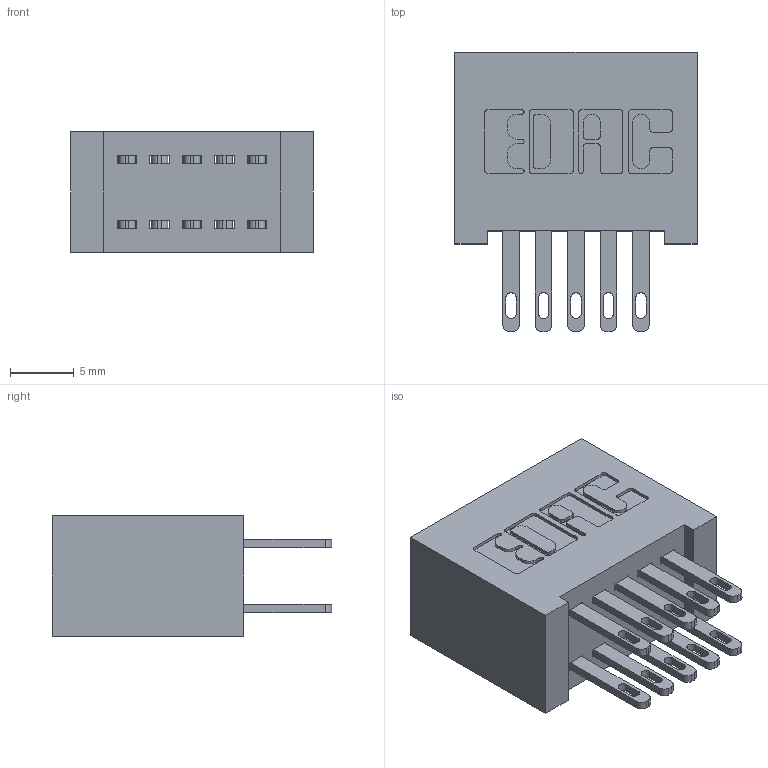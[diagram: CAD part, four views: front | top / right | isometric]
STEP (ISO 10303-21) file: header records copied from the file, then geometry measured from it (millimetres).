
FILE_DESCRIPTION (( 'STEP AP203' ), '1' );
FILE_NAME ('892-010-500-201.STEP', '2020-09-21T12:49:18', ( '' ), ( '' ), 'SwSTEP 2.0', 'SolidWorks 2020', '' );
FILE_SCHEMA (( 'CONFIG_CONTROL_DESIGN' ));
Length unit declared in the file: inch
Products named in the file (3): 842 Part_Lugless; 892-010-500-201; 345-292-001_345-293-100
Assembly tree (11 placements, depth 2):
  892-010-500-201
    842 Part_Lugless
    345-292-001_345-293-100  x10
Bounding box: 18.95 x 21.85 x 9.4 mm (x, y, z)
Volume: 1997.4 mm3; surface area: 2881.6 mm2
Topology: 11 solids, 11 shells, 582 faces, 1745 edges, 1162 vertices
Faces by surface type: plane 362, cylinder 220
Entity records: 7523 total; most frequent: CARTESIAN_POINT 1286, ORIENTED_EDGE 1222, DIRECTION 1159, EDGE_CURVE 611, LINE 487, VECTOR 487, VERTEX_POINT 406, AXIS2_PLACEMENT_3D 336
